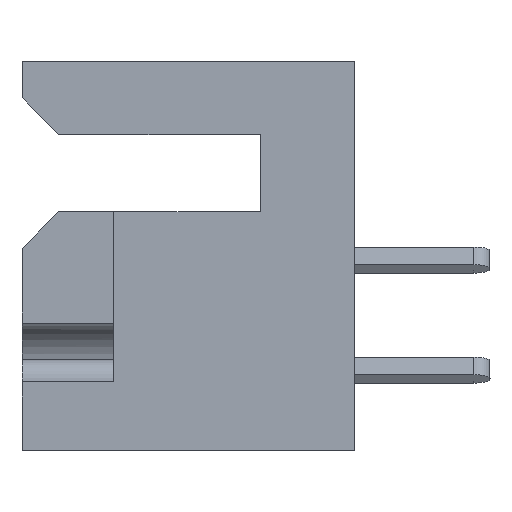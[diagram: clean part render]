
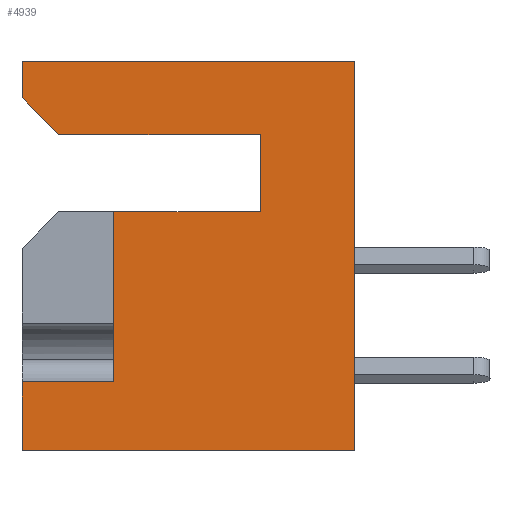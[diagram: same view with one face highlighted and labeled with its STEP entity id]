
A CAD part, left-side view. The second image highlights one B-rep face of the part: STEP entity #4939.
In plain terms, the highlighted planar face has unit normal (-1, 0, 0).
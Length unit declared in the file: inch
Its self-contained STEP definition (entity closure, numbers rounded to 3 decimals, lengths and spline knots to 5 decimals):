
#283 = DIRECTION ( 'NONE',  ( 0., -0.707, -0.707 ) ) ;
#798 = DIRECTION ( 'NONE',  ( 0., 0., 1. ) ) ;
#1290 = VECTOR ( 'NONE', #15636, 39.37008 ) ;
#1819 = CARTESIAN_POINT ( 'NONE',  ( 0., 0.453, -0.437 ) ) ;
#2696 = VERTEX_POINT ( 'NONE', #6733 ) ;
#2924 = VERTEX_POINT ( 'NONE', #20525 ) ;
#3061 = VECTOR ( 'NONE', #9394, 39.37008 ) ;
#3146 = CARTESIAN_POINT ( 'NONE',  ( 0., 0.328, -0.205 ) ) ;
#4353 = LINE ( 'NONE', #27142, #6080 ) ;
#4423 = VERTEX_POINT ( 'NONE', #5842 ) ;
#4472 = CARTESIAN_POINT ( 'NONE',  ( 0., 0.453, 0. ) ) ;
#4569 = DIRECTION ( 'NONE',  ( 0., 0., 1. ) ) ;
#4612 = CARTESIAN_POINT ( 'NONE',  ( 0., 0., 0. ) ) ;
#4939 = ADVANCED_FACE ( 'NONE', ( #5040 ), #23081, .F. ) ;
#5040 = FACE_OUTER_BOUND ( 'NONE', #15413, .T. ) ;
#5553 = CARTESIAN_POINT ( 'NONE',  ( 0., 0., 0. ) ) ;
#5842 = CARTESIAN_POINT ( 'NONE',  ( 0., 0.453, -0.531 ) ) ;
#6080 = VECTOR ( 'NONE', #26861, 39.37008 ) ;
#6733 = CARTESIAN_POINT ( 'NONE',  ( 0., 0., -0.531 ) ) ;
#6756 = DIRECTION ( 'NONE',  ( 0., 0., 1. ) ) ;
#7185 = VERTEX_POINT ( 'NONE', #17552 ) ;
#7797 = CARTESIAN_POINT ( 'NONE',  ( 0., 0.328, -0.437 ) ) ;
#7911 = LINE ( 'NONE', #4472, #20330 ) ;
#8434 = ORIENTED_EDGE ( 'NONE', *, *, #18651, .F. ) ;
#8770 = ORIENTED_EDGE ( 'NONE', *, *, #19127, .T. ) ;
#8904 = LINE ( 'NONE', #14543, #1290 ) ;
#9213 = CARTESIAN_POINT ( 'NONE',  ( 0., 0.453, 0. ) ) ;
#9386 = VERTEX_POINT ( 'NONE', #4612 ) ;
#9394 = DIRECTION ( 'NONE',  ( 0., -1., 0. ) ) ;
#9499 = DIRECTION ( 'NONE',  ( 0., 0., 1. ) ) ;
#9843 = DIRECTION ( 'NONE',  ( 1., 0., 0. ) ) ;
#9870 = VECTOR ( 'NONE', #23114, 39.37008 ) ;
#10587 = DIRECTION ( 'NONE',  ( 0., -1., 0. ) ) ;
#10644 = EDGE_CURVE ( 'NONE', #4423, #13407, #7911, .T. ) ;
#10730 = EDGE_CURVE ( 'NONE', #2924, #9386, #19660, .T. ) ;
#10823 = VECTOR ( 'NONE', #6756, 39.37008 ) ;
#11788 = CARTESIAN_POINT ( 'NONE',  ( 0., 0.453, 0. ) ) ;
#12136 = CARTESIAN_POINT ( 'NONE',  ( 0., 0.328, -0.437 ) ) ;
#12613 = LINE ( 'NONE', #9213, #27458 ) ;
#13407 = VERTEX_POINT ( 'NONE', #1819 ) ;
#13479 = EDGE_CURVE ( 'NONE', #7185, #19139, #21550, .T. ) ;
#14052 = VECTOR ( 'NONE', #19276, 39.37008 ) ;
#14543 = CARTESIAN_POINT ( 'NONE',  ( 0., 0.328, -0.205 ) ) ;
#14770 = ORIENTED_EDGE ( 'NONE', *, *, #10644, .F. ) ;
#14789 = ORIENTED_EDGE ( 'NONE', *, *, #28544, .T. ) ;
#14821 = AXIS2_PLACEMENT_3D ( 'NONE', #11788, #9843, #22690 ) ;
#14907 = CARTESIAN_POINT ( 'NONE',  ( 0., 0.128, -0.1 ) ) ;
#15143 = ORIENTED_EDGE ( 'NONE', *, *, #19432, .F. ) ;
#15413 = EDGE_LOOP ( 'NONE', ( #8770, #14770, #17396, #19578, #20022, #22683, #14789, #15143, #28556, #19622, #8434 ) ) ;
#15442 = CARTESIAN_POINT ( 'NONE',  ( 0., 0.453, -0.05 ) ) ;
#15636 = DIRECTION ( 'NONE',  ( 0., 0., 1. ) ) ;
#15748 = CARTESIAN_POINT ( 'NONE',  ( 0., 0.453, 0. ) ) ;
#16082 = LINE ( 'NONE', #5553, #23011 ) ;
#17075 = CARTESIAN_POINT ( 'NONE',  ( 0., 0.453, -0.531 ) ) ;
#17396 = ORIENTED_EDGE ( 'NONE', *, *, #23355, .T. ) ;
#17552 = CARTESIAN_POINT ( 'NONE',  ( 0., 0.128, -0.205 ) ) ;
#18505 = VERTEX_POINT ( 'NONE', #3146 ) ;
#18626 = CARTESIAN_POINT ( 'NONE',  ( 0., 0.403, -0.1 ) ) ;
#18641 = VECTOR ( 'NONE', #283, 39.37008 ) ;
#18651 = EDGE_CURVE ( 'NONE', #18832, #18505, #8904, .T. ) ;
#18832 = VERTEX_POINT ( 'NONE', #12136 ) ;
#19127 = EDGE_CURVE ( 'NONE', #18832, #13407, #23037, .T. ) ;
#19139 = VERTEX_POINT ( 'NONE', #14907 ) ;
#19276 = DIRECTION ( 'NONE',  ( 0., 1., 0. ) ) ;
#19385 = EDGE_CURVE ( 'NONE', #21758, #2924, #12613, .T. ) ;
#19432 = EDGE_CURVE ( 'NONE', #19139, #20770, #4353, .T. ) ;
#19479 = EDGE_CURVE ( 'NONE', #2696, #9386, #16082, .T. ) ;
#19578 = ORIENTED_EDGE ( 'NONE', *, *, #19479, .T. ) ;
#19586 = EDGE_CURVE ( 'NONE', #7185, #18505, #19904, .T. ) ;
#19622 = ORIENTED_EDGE ( 'NONE', *, *, #19586, .T. ) ;
#19660 = LINE ( 'NONE', #15748, #3061 ) ;
#19904 = LINE ( 'NONE', #27511, #9870 ) ;
#20022 = ORIENTED_EDGE ( 'NONE', *, *, #10730, .F. ) ;
#20330 = VECTOR ( 'NONE', #4569, 39.37008 ) ;
#20525 = CARTESIAN_POINT ( 'NONE',  ( 0., 0.453, 0. ) ) ;
#20770 = VERTEX_POINT ( 'NONE', #18626 ) ;
#21550 = LINE ( 'NONE', #28570, #10823 ) ;
#21758 = VERTEX_POINT ( 'NONE', #15442 ) ;
#22109 = CARTESIAN_POINT ( 'NONE',  ( 0., 0.403, -0.1 ) ) ;
#22683 = ORIENTED_EDGE ( 'NONE', *, *, #19385, .F. ) ;
#22690 = DIRECTION ( 'NONE',  ( 0., 0., -1. ) ) ;
#23011 = VECTOR ( 'NONE', #798, 39.37008 ) ;
#23037 = LINE ( 'NONE', #7797, #14052 ) ;
#23081 = PLANE ( 'NONE',  #14821 ) ;
#23114 = DIRECTION ( 'NONE',  ( 0., 1., 0. ) ) ;
#23355 = EDGE_CURVE ( 'NONE', #4423, #2696, #27060, .T. ) ;
#25006 = VECTOR ( 'NONE', #10587, 39.37008 ) ;
#26212 = LINE ( 'NONE', #22109, #18641 ) ;
#26861 = DIRECTION ( 'NONE',  ( 0., 1., 0. ) ) ;
#27060 = LINE ( 'NONE', #17075, #25006 ) ;
#27142 = CARTESIAN_POINT ( 'NONE',  ( 0., 0.128, -0.1 ) ) ;
#27458 = VECTOR ( 'NONE', #9499, 39.37008 ) ;
#27511 = CARTESIAN_POINT ( 'NONE',  ( 0., 0.128, -0.205 ) ) ;
#28544 = EDGE_CURVE ( 'NONE', #21758, #20770, #26212, .T. ) ;
#28556 = ORIENTED_EDGE ( 'NONE', *, *, #13479, .F. ) ;
#28570 = CARTESIAN_POINT ( 'NONE',  ( 0., 0.128, -0.1 ) ) ;
